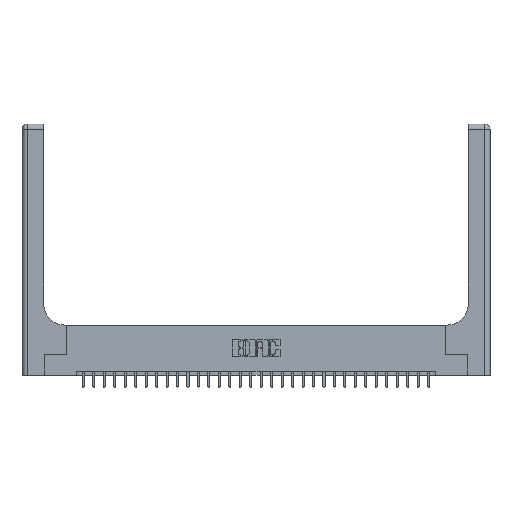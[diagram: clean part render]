
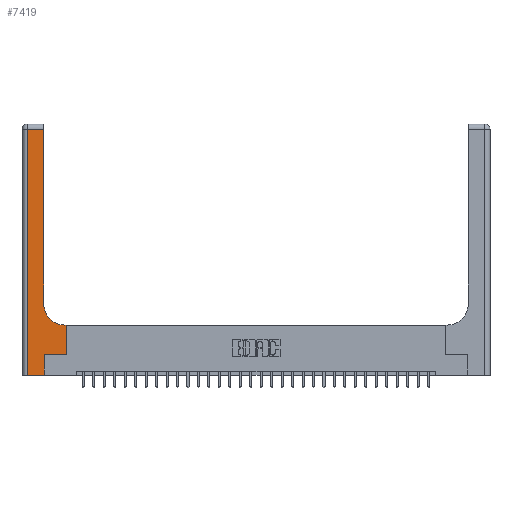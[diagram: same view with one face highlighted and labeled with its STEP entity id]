
A CAD part, top view. The second image highlights one B-rep face of the part: STEP entity #7419.
In plain terms, the highlighted planar face has unit normal (0, 0, 1).
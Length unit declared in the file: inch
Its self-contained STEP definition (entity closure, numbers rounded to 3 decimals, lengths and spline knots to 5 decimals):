
#126 = DIRECTION ( 'NONE',  ( 0., -1., 0. ) ) ;
#329 = DIRECTION ( 'NONE',  ( -1., 0., 0. ) ) ;
#450 = DIRECTION ( 'NONE',  ( -1., 0., 0. ) ) ;
#1809 = VERTEX_POINT ( 'NONE', #16210 ) ;
#2082 = DIRECTION ( 'NONE',  ( 1., 0., 0. ) ) ;
#2369 = CARTESIAN_POINT ( 'NONE',  ( 0.26, 2.94, 0.37 ) ) ;
#3080 = CARTESIAN_POINT ( 'NONE',  ( 0., 2.94, 0.37 ) ) ;
#3618 = VECTOR ( 'NONE', #126, 39.37008 ) ;
#3772 = EDGE_CURVE ( 'NONE', #24079, #24803, #24612, .T. ) ;
#3817 = PLANE ( 'NONE',  #13864 ) ;
#3842 = DIRECTION ( 'NONE',  ( 0., 0., -1. ) ) ;
#4025 = CARTESIAN_POINT ( 'NONE',  ( 0.528, 0.6, 0.37 ) ) ;
#4237 = VECTOR ( 'NONE', #329, 39.37008 ) ;
#4556 = DIRECTION ( 'NONE',  ( 1., 0., 0. ) ) ;
#4657 = LINE ( 'NONE', #24572, #3618 ) ;
#5131 = DIRECTION ( 'NONE',  ( -1., 0., 0. ) ) ;
#5213 = DIRECTION ( 'NONE',  ( 0., 1., 0. ) ) ;
#5358 = LINE ( 'NONE', #27885, #23562 ) ;
#5382 = CARTESIAN_POINT ( 'NONE',  ( 0., 0., 0.37 ) ) ;
#5441 = CARTESIAN_POINT ( 'NONE',  ( 0.51, 0.6, 0.37 ) ) ;
#5575 = CARTESIAN_POINT ( 'NONE',  ( 0.06, 2.94, 0.37 ) ) ;
#5593 = CARTESIAN_POINT ( 'NONE',  ( 0.26, 3., 0.37 ) ) ;
#6007 = FACE_OUTER_BOUND ( 'NONE', #13687, .T. ) ;
#6902 = CARTESIAN_POINT ( 'NONE',  ( 0.26, 0.6, 0.37 ) ) ;
#7419 = ADVANCED_FACE ( 'NONE', ( #6007 ), #3817, .F. ) ;
#7699 = ORIENTED_EDGE ( 'NONE', *, *, #19054, .T. ) ;
#7710 = LINE ( 'NONE', #5382, #25652 ) ;
#8274 = ORIENTED_EDGE ( 'NONE', *, *, #21294, .T. ) ;
#8402 = AXIS2_PLACEMENT_3D ( 'NONE', #13064, #3842, #2082 ) ;
#9095 = CARTESIAN_POINT ( 'NONE',  ( 0.265, 0.25, 0.37 ) ) ;
#9213 = EDGE_CURVE ( 'NONE', #22151, #1809, #4657, .T. ) ;
#10091 = DIRECTION ( 'NONE',  ( 0., 1., 0. ) ) ;
#10191 = DIRECTION ( 'NONE',  ( 1., 0., 0. ) ) ;
#10842 = CARTESIAN_POINT ( 'NONE',  ( 0.528, 0.25, 0.37 ) ) ;
#10969 = VERTEX_POINT ( 'NONE', #2369 ) ;
#11131 = DIRECTION ( 'NONE',  ( 0., 0., -1. ) ) ;
#11236 = CARTESIAN_POINT ( 'NONE',  ( 0.265, 0.25, 0.37 ) ) ;
#11378 = VERTEX_POINT ( 'NONE', #19767 ) ;
#13053 = ORIENTED_EDGE ( 'NONE', *, *, #25267, .T. ) ;
#13064 = CARTESIAN_POINT ( 'NONE',  ( 0.51, 0.85, 0.37 ) ) ;
#13687 = EDGE_LOOP ( 'NONE', ( #13734, #21307, #14598, #7699, #13053, #24480, #8274, #28349, #17019 ) ) ;
#13734 = ORIENTED_EDGE ( 'NONE', *, *, #21317, .T. ) ;
#13846 = EDGE_CURVE ( 'NONE', #22650, #14126, #22278, .T. ) ;
#13864 = AXIS2_PLACEMENT_3D ( 'NONE', #22552, #11131, #450 ) ;
#14126 = VERTEX_POINT ( 'NONE', #5441 ) ;
#14598 = ORIENTED_EDGE ( 'NONE', *, *, #9213, .T. ) ;
#14898 = EDGE_CURVE ( 'NONE', #14126, #20235, #22447, .T. ) ;
#16210 = CARTESIAN_POINT ( 'NONE',  ( 0.06, 0., 0.37 ) ) ;
#16459 = LINE ( 'NONE', #5593, #23808 ) ;
#17019 = ORIENTED_EDGE ( 'NONE', *, *, #14898, .T. ) ;
#17884 = CARTESIAN_POINT ( 'NONE',  ( 0.26, 0.85, 0.37 ) ) ;
#19054 = EDGE_CURVE ( 'NONE', #1809, #11378, #7710, .T. ) ;
#19454 = CARTESIAN_POINT ( 'NONE',  ( 0.265, 0., 0.37 ) ) ;
#19767 = CARTESIAN_POINT ( 'NONE',  ( 0.265, 0., 0.37 ) ) ;
#20235 = VERTEX_POINT ( 'NONE', #17884 ) ;
#20237 = VECTOR ( 'NONE', #5131, 39.37008 ) ;
#21155 = VECTOR ( 'NONE', #10091, 39.37008 ) ;
#21294 = EDGE_CURVE ( 'NONE', #24803, #22650, #5358, .T. ) ;
#21307 = ORIENTED_EDGE ( 'NONE', *, *, #25075, .T. ) ;
#21317 = EDGE_CURVE ( 'NONE', #20235, #10969, #16459, .T. ) ;
#22151 = VERTEX_POINT ( 'NONE', #5575 ) ;
#22278 = LINE ( 'NONE', #6902, #4237 ) ;
#22447 = CIRCLE ( 'NONE', #8402, 0.25 ) ;
#22552 = CARTESIAN_POINT ( 'NONE',  ( 0., 3., 0.37 ) ) ;
#22650 = VERTEX_POINT ( 'NONE', #4025 ) ;
#23457 = DIRECTION ( 'NONE',  ( 0., 1., 0. ) ) ;
#23562 = VECTOR ( 'NONE', #5213, 39.37008 ) ;
#23621 = VECTOR ( 'NONE', #4556, 39.37008 ) ;
#23808 = VECTOR ( 'NONE', #23457, 39.37008 ) ;
#24079 = VERTEX_POINT ( 'NONE', #11236 ) ;
#24480 = ORIENTED_EDGE ( 'NONE', *, *, #3772, .T. ) ;
#24572 = CARTESIAN_POINT ( 'NONE',  ( 0.06, 3., 0.37 ) ) ;
#24612 = LINE ( 'NONE', #9095, #23621 ) ;
#24803 = VERTEX_POINT ( 'NONE', #10842 ) ;
#25075 = EDGE_CURVE ( 'NONE', #10969, #22151, #25182, .T. ) ;
#25182 = LINE ( 'NONE', #3080, #20237 ) ;
#25267 = EDGE_CURVE ( 'NONE', #11378, #24079, #28225, .T. ) ;
#25652 = VECTOR ( 'NONE', #10191, 39.37008 ) ;
#27885 = CARTESIAN_POINT ( 'NONE',  ( 0.528, 0.25, 0.37 ) ) ;
#28225 = LINE ( 'NONE', #19454, #21155 ) ;
#28349 = ORIENTED_EDGE ( 'NONE', *, *, #13846, .T. ) ;
